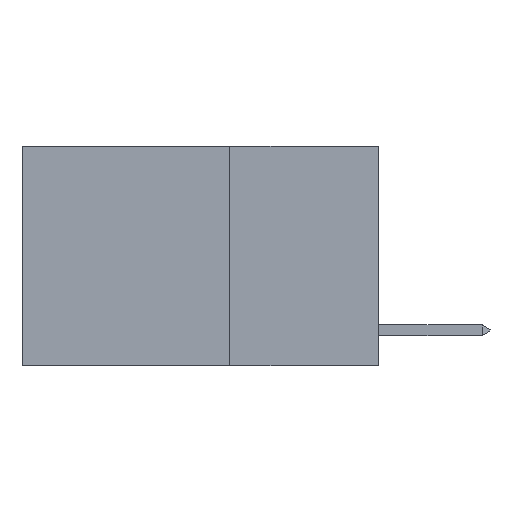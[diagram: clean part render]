
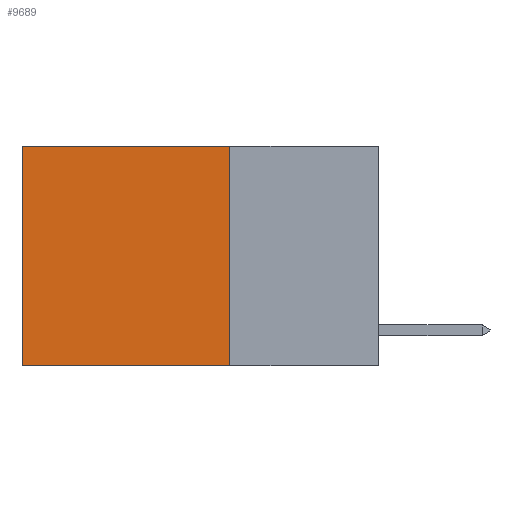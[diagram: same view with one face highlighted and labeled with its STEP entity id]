
A CAD part, left-side view. The second image highlights one B-rep face of the part: STEP entity #9689.
In plain terms, the highlighted planar face has unit normal (-1, 0, 0).
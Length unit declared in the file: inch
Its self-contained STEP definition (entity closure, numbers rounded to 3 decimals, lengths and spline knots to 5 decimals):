
#918 = CARTESIAN_POINT ( 'NONE',  ( 0.2625, 0.6, 0. ) ) ;
#1272 = VECTOR ( 'NONE', #6761, 39.37008 ) ;
#1285 = LINE ( 'NONE', #8818, #7986 ) ;
#1350 = EDGE_CURVE ( 'NONE', #13843, #15762, #1285, .T. ) ;
#1411 = ORIENTED_EDGE ( 'NONE', *, *, #1350, .F. ) ;
#1535 = LINE ( 'NONE', #5999, #4692 ) ;
#1642 = EDGE_CURVE ( 'NONE', #15762, #3325, #8375, .T. ) ;
#1880 = DIRECTION ( 'NONE',  ( 0., 1., 0. ) ) ;
#2045 = VERTEX_POINT ( 'NONE', #918 ) ;
#2576 = ORIENTED_EDGE ( 'NONE', *, *, #15165, .T. ) ;
#3325 = VERTEX_POINT ( 'NONE', #16775 ) ;
#4692 = VECTOR ( 'NONE', #12522, 39.37008 ) ;
#4875 = CARTESIAN_POINT ( 'NONE',  ( 0.2625, 0.25, 0. ) ) ;
#5999 = CARTESIAN_POINT ( 'NONE',  ( 0.2625, 0.6, 0. ) ) ;
#6226 = DIRECTION ( 'NONE',  ( 0., 0., -1. ) ) ;
#6761 = DIRECTION ( 'NONE',  ( 0., 1., 0. ) ) ;
#7082 = EDGE_CURVE ( 'NONE', #13843, #2045, #14341, .T. ) ;
#7482 = PLANE ( 'NONE',  #8627 ) ;
#7986 = VECTOR ( 'NONE', #12817, 39.37008 ) ;
#8375 = LINE ( 'NONE', #15993, #1272 ) ;
#8627 = AXIS2_PLACEMENT_3D ( 'NONE', #4875, #14123, #6226 ) ;
#8818 = CARTESIAN_POINT ( 'NONE',  ( 0.2625, 0.25, 0. ) ) ;
#9689 = ADVANCED_FACE ( 'NONE', ( #16672 ), #7482, .F. ) ;
#9706 = CARTESIAN_POINT ( 'NONE',  ( 0.2625, 0.25, 0. ) ) ;
#11177 = CARTESIAN_POINT ( 'NONE',  ( 0.2625, 0.25, 0. ) ) ;
#12522 = DIRECTION ( 'NONE',  ( 0., 0., -1. ) ) ;
#12817 = DIRECTION ( 'NONE',  ( 0., 0., -1. ) ) ;
#13549 = ORIENTED_EDGE ( 'NONE', *, *, #7082, .T. ) ;
#13843 = VERTEX_POINT ( 'NONE', #9706 ) ;
#13928 = VECTOR ( 'NONE', #1880, 39.37008 ) ;
#14123 = DIRECTION ( 'NONE',  ( 1., 0., 0. ) ) ;
#14341 = LINE ( 'NONE', #11177, #13928 ) ;
#15165 = EDGE_CURVE ( 'NONE', #2045, #3325, #1535, .T. ) ;
#15176 = CARTESIAN_POINT ( 'NONE',  ( 0.2625, 0.25, -0.37 ) ) ;
#15182 = EDGE_LOOP ( 'NONE', ( #2576, #15835, #1411, #13549 ) ) ;
#15762 = VERTEX_POINT ( 'NONE', #15176 ) ;
#15835 = ORIENTED_EDGE ( 'NONE', *, *, #1642, .F. ) ;
#15993 = CARTESIAN_POINT ( 'NONE',  ( 0.2625, 0.25, -0.37 ) ) ;
#16672 = FACE_OUTER_BOUND ( 'NONE', #15182, .T. ) ;
#16775 = CARTESIAN_POINT ( 'NONE',  ( 0.2625, 0.6, -0.37 ) ) ;
